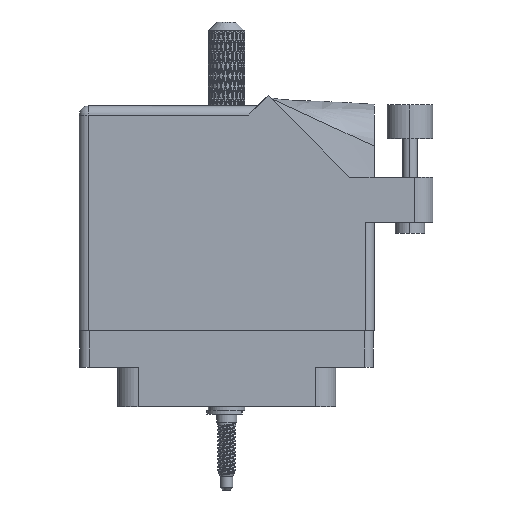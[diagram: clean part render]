
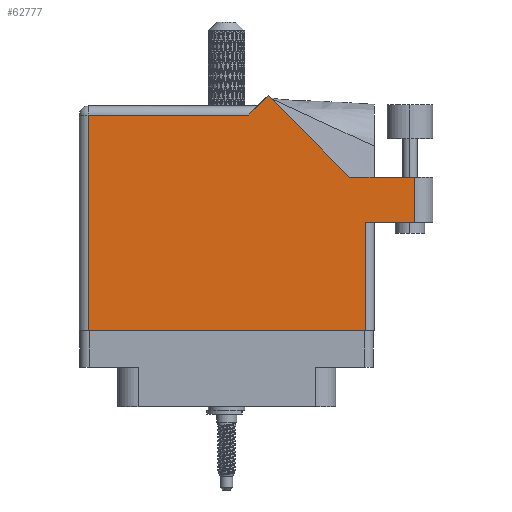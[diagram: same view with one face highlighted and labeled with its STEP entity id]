
A CAD part, front view. The second image highlights one B-rep face of the part: STEP entity #62777.
In plain terms, the highlighted face is planar.
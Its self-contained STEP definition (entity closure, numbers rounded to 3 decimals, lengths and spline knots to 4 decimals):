
#64 = VERTEX_POINT ( 'NONE', #50408 ) ;
#226 = ORIENTED_EDGE ( 'NONE', *, *, #41317, .T. ) ;
#2194 = VERTEX_POINT ( 'NONE', #83624 ) ;
#5014 = EDGE_CURVE ( 'NONE', #64, #8271, #38981, .T. ) ;
#7256 = CARTESIAN_POINT ( 'NONE',  ( -0.943, -0.1, 0.455 ) ) ;
#8271 = VERTEX_POINT ( 'NONE', #51999 ) ;
#10557 = VECTOR ( 'NONE', #93321, 39.3701 ) ;
#12264 = CARTESIAN_POINT ( 'NONE',  ( 1.405, 0.944, 0.455 ) ) ;
#12987 = ORIENTED_EDGE ( 'NONE', *, *, #5014, .T. ) ;
#13621 = AXIS2_PLACEMENT_3D ( 'NONE', #21104, #78237, #87151 ) ;
#14250 = VECTOR ( 'NONE', #98389, 39.3701 ) ;
#14306 = EDGE_CURVE ( 'NONE', #90368, #96962, #24049, .T. ) ;
#15541 = VECTOR ( 'NONE', #66893, 39.3701 ) ;
#18999 = CARTESIAN_POINT ( 'NONE',  ( 0.943, -0.1, 0.455 ) ) ;
#21104 = CARTESIAN_POINT ( 'NONE',  ( -1.005, 1.43, 0.455 ) ) ;
#21668 = EDGE_CURVE ( 'NONE', #78872, #64, #92202, .T. ) ;
#24049 = LINE ( 'NONE', #35311, #62374 ) ;
#25813 = CARTESIAN_POINT ( 'NONE',  ( 0.2827, 1.5007, 0.455 ) ) ;
#25841 = LINE ( 'NONE', #12264, #10557 ) ;
#27280 = LINE ( 'NONE', #81485, #29904 ) ;
#29389 = CARTESIAN_POINT ( 'NONE',  ( 0.15, 1.368, 0.455 ) ) ;
#29904 = VECTOR ( 'NONE', #47332, 39.3701 ) ;
#30101 = PLANE ( 'NONE',  #13621 ) ;
#32990 = EDGE_CURVE ( 'NONE', #2194, #79367, #98200, .T. ) ;
#35311 = CARTESIAN_POINT ( 'NONE',  ( 0.212, 1.43, 0.455 ) ) ;
#36377 = CARTESIAN_POINT ( 'NONE',  ( 0.8394, 0.944, 0.455 ) ) ;
#37146 = VECTOR ( 'NONE', #101595, 39.3701 ) ;
#37712 = CARTESIAN_POINT ( 'NONE',  ( 1.28, 0.944, 0.455 ) ) ;
#38981 = LINE ( 'NONE', #37712, #58144 ) ;
#40689 = CARTESIAN_POINT ( 'NONE',  ( 0.8394, 0.944, 0.455 ) ) ;
#41317 = EDGE_CURVE ( 'NONE', #79367, #78872, #27280, .T. ) ;
#42136 = VERTEX_POINT ( 'NONE', #40689 ) ;
#42228 = EDGE_CURVE ( 'NONE', #8271, #42136, #25841, .T. ) ;
#43053 = FACE_OUTER_BOUND ( 'NONE', #76869, .T. ) ;
#47332 = DIRECTION ( 'NONE',  ( 0., 1., 0. ) ) ;
#47800 = CARTESIAN_POINT ( 'NONE',  ( -1.005, -0.1, 0.455 ) ) ;
#48076 = DIRECTION ( 'NONE',  ( 0., -1., 0. ) ) ;
#48520 = VECTOR ( 'NONE', #104752, 39.3701 ) ;
#48626 = CARTESIAN_POINT ( 'NONE',  ( 0.943, 0.637, 0.455 ) ) ;
#50408 = CARTESIAN_POINT ( 'NONE',  ( 1.28, 0.637, 0.455 ) ) ;
#51071 = DIRECTION ( 'NONE',  ( -0.707, -0.707, 0. ) ) ;
#51638 = EDGE_CURVE ( 'NONE', #56541, #2194, #79981, .T. ) ;
#51999 = CARTESIAN_POINT ( 'NONE',  ( 1.28, 0.944, 0.455 ) ) ;
#55237 = DIRECTION ( 'NONE',  ( 0., 1., 0. ) ) ;
#55362 = EDGE_CURVE ( 'NONE', #96962, #56541, #103719, .T. ) ;
#55456 = ORIENTED_EDGE ( 'NONE', *, *, #21668, .T. ) ;
#56541 = VERTEX_POINT ( 'NONE', #78559 ) ;
#58144 = VECTOR ( 'NONE', #55237, 39.3701 ) ;
#58786 = CARTESIAN_POINT ( 'NONE',  ( -1.005, 1.368, 0.455 ) ) ;
#60275 = ORIENTED_EDGE ( 'NONE', *, *, #51638, .T. ) ;
#62374 = VECTOR ( 'NONE', #51071, 39.3701 ) ;
#62777 = ADVANCED_FACE ( 'NONE', ( #43053 ), #30101, .F. ) ;
#66893 = DIRECTION ( 'NONE',  ( -1., 0., 0. ) ) ;
#67557 = ORIENTED_EDGE ( 'NONE', *, *, #14306, .T. ) ;
#72298 = VECTOR ( 'NONE', #48076, 39.3701 ) ;
#73621 = ORIENTED_EDGE ( 'NONE', *, *, #96248, .T. ) ;
#76869 = EDGE_LOOP ( 'NONE', ( #55456, #12987, #94553, #73621, #67557, #94962, #60275, #90867, #226 ) ) ;
#78237 = DIRECTION ( 'NONE',  ( 0., 0., -1. ) ) ;
#78559 = CARTESIAN_POINT ( 'NONE',  ( -0.943, 1.368, 0.455 ) ) ;
#78872 = VERTEX_POINT ( 'NONE', #48626 ) ;
#79367 = VERTEX_POINT ( 'NONE', #18999 ) ;
#79981 = LINE ( 'NONE', #7256, #72298 ) ;
#81485 = CARTESIAN_POINT ( 'NONE',  ( 0.943, 0.637, 0.455 ) ) ;
#82307 = CARTESIAN_POINT ( 'NONE',  ( 1.005, 0.637, 0.455 ) ) ;
#83624 = CARTESIAN_POINT ( 'NONE',  ( -0.943, -0.1, 0.455 ) ) ;
#87151 = DIRECTION ( 'NONE',  ( -1., 0., 0. ) ) ;
#90368 = VERTEX_POINT ( 'NONE', #25813 ) ;
#90867 = ORIENTED_EDGE ( 'NONE', *, *, #32990, .T. ) ;
#92202 = LINE ( 'NONE', #82307, #14250 ) ;
#93321 = DIRECTION ( 'NONE',  ( -1., 0., 0. ) ) ;
#94553 = ORIENTED_EDGE ( 'NONE', *, *, #42228, .T. ) ;
#94962 = ORIENTED_EDGE ( 'NONE', *, *, #55362, .T. ) ;
#96248 = EDGE_CURVE ( 'NONE', #42136, #90368, #102219, .T. ) ;
#96962 = VERTEX_POINT ( 'NONE', #29389 ) ;
#98200 = LINE ( 'NONE', #47800, #48520 ) ;
#98389 = DIRECTION ( 'NONE',  ( 1., 0., 0. ) ) ;
#101595 = DIRECTION ( 'NONE',  ( -0.707, 0.707, 0. ) ) ;
#102219 = LINE ( 'NONE', #36377, #37146 ) ;
#103719 = LINE ( 'NONE', #58786, #15541 ) ;
#104752 = DIRECTION ( 'NONE',  ( 1., 0., 0. ) ) ;
